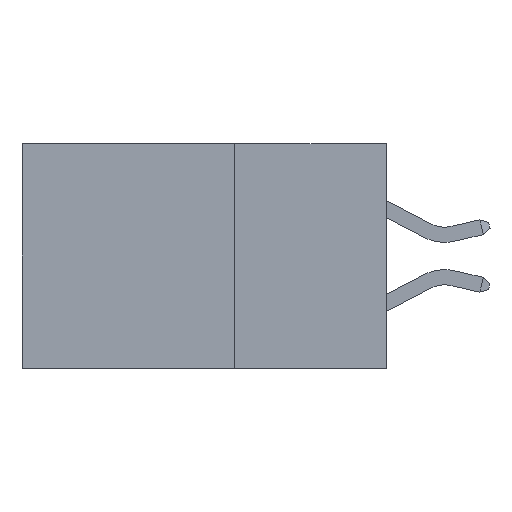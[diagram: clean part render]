
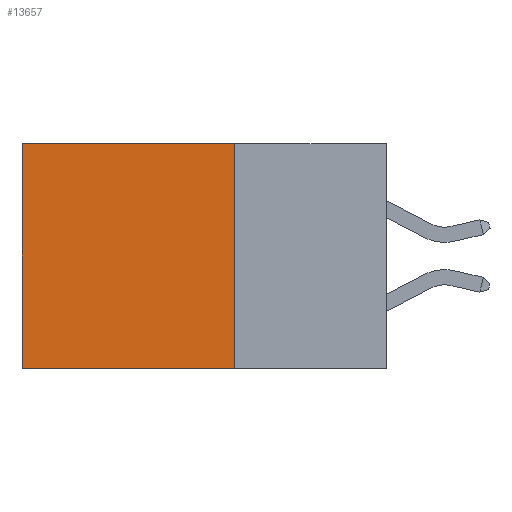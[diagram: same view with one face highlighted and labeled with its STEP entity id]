
A CAD part, left-side view. The second image highlights one B-rep face of the part: STEP entity #13657.
In plain terms, the highlighted planar face has unit normal (-1, 0, 0).
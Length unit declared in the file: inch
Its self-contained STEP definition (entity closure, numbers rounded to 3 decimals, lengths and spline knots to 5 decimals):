
#69 = PLANE ( 'NONE',  #8878 ) ;
#782 = DIRECTION ( 'NONE',  ( 0., 1., 0. ) ) ;
#1175 = EDGE_CURVE ( 'NONE', #14753, #5438, #5956, .T. ) ;
#1271 = DIRECTION ( 'NONE',  ( 0., 0., -1. ) ) ;
#1415 = LINE ( 'NONE', #2628, #7357 ) ;
#1732 = CARTESIAN_POINT ( 'NONE',  ( 0.298, 0.6, 0. ) ) ;
#2267 = CARTESIAN_POINT ( 'NONE',  ( 0.298, 0.6, 0. ) ) ;
#2435 = VECTOR ( 'NONE', #4271, 39.37008 ) ;
#2535 = EDGE_CURVE ( 'NONE', #14753, #14203, #3693, .T. ) ;
#2628 = CARTESIAN_POINT ( 'NONE',  ( 0.298, 0.25, -0.37 ) ) ;
#2665 = CARTESIAN_POINT ( 'NONE',  ( 0.298, 0.6, -0.37 ) ) ;
#3315 = VECTOR ( 'NONE', #782, 39.37008 ) ;
#3693 = LINE ( 'NONE', #13768, #3315 ) ;
#4138 = LINE ( 'NONE', #1732, #6906 ) ;
#4271 = DIRECTION ( 'NONE',  ( 0., 0., -1. ) ) ;
#4456 = EDGE_LOOP ( 'NONE', ( #8568, #8555, #8433, #9674 ) ) ;
#4572 = CARTESIAN_POINT ( 'NONE',  ( 0.298, 0.25, 0. ) ) ;
#5002 = VERTEX_POINT ( 'NONE', #2665 ) ;
#5438 = VERTEX_POINT ( 'NONE', #14344 ) ;
#5956 = LINE ( 'NONE', #4572, #2435 ) ;
#6431 = DIRECTION ( 'NONE',  ( 0., 0., -1. ) ) ;
#6906 = VECTOR ( 'NONE', #6431, 39.37008 ) ;
#7357 = VECTOR ( 'NONE', #12175, 39.37008 ) ;
#8012 = EDGE_CURVE ( 'NONE', #14203, #5002, #4138, .T. ) ;
#8197 = CARTESIAN_POINT ( 'NONE',  ( 0.298, 0.25, 0. ) ) ;
#8383 = DIRECTION ( 'NONE',  ( 1., 0., 0. ) ) ;
#8433 = ORIENTED_EDGE ( 'NONE', *, *, #1175, .F. ) ;
#8555 = ORIENTED_EDGE ( 'NONE', *, *, #12519, .F. ) ;
#8568 = ORIENTED_EDGE ( 'NONE', *, *, #8012, .T. ) ;
#8878 = AXIS2_PLACEMENT_3D ( 'NONE', #11943, #8383, #1271 ) ;
#9674 = ORIENTED_EDGE ( 'NONE', *, *, #2535, .T. ) ;
#11109 = FACE_OUTER_BOUND ( 'NONE', #4456, .T. ) ;
#11943 = CARTESIAN_POINT ( 'NONE',  ( 0.298, 0.25, 0. ) ) ;
#12175 = DIRECTION ( 'NONE',  ( 0., 1., 0. ) ) ;
#12519 = EDGE_CURVE ( 'NONE', #5438, #5002, #1415, .T. ) ;
#13657 = ADVANCED_FACE ( 'NONE', ( #11109 ), #69, .F. ) ;
#13768 = CARTESIAN_POINT ( 'NONE',  ( 0.298, 0.25, 0. ) ) ;
#14203 = VERTEX_POINT ( 'NONE', #2267 ) ;
#14344 = CARTESIAN_POINT ( 'NONE',  ( 0.298, 0.25, -0.37 ) ) ;
#14753 = VERTEX_POINT ( 'NONE', #8197 ) ;
